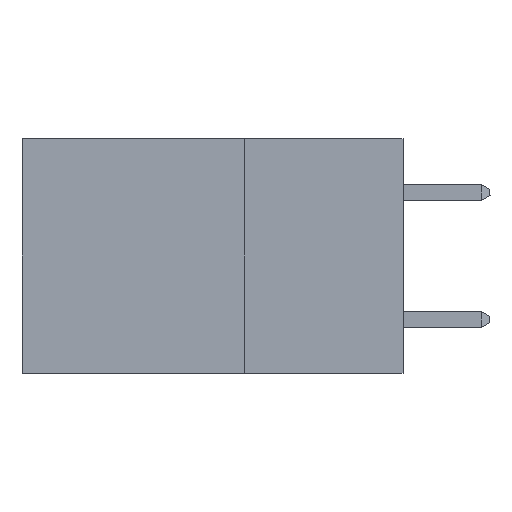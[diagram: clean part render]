
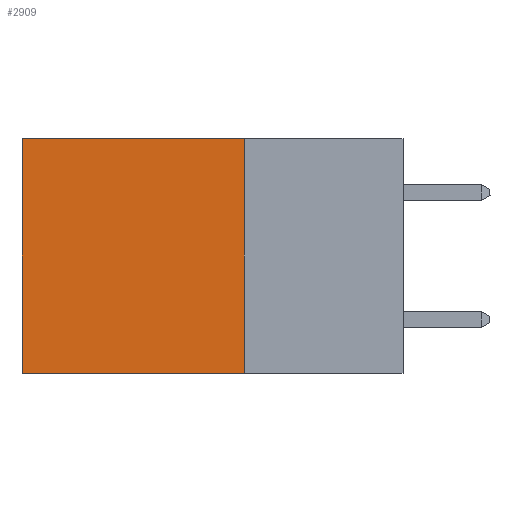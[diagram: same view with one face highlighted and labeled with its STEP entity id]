
A CAD part, left-side view. The second image highlights one B-rep face of the part: STEP entity #2909.
In plain terms, the highlighted planar face has unit normal (-1, 0, 0).
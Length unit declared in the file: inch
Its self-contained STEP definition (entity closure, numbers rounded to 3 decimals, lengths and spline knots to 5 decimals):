
#186 = DIRECTION ( 'NONE',  ( 0., 1., 0. ) ) ;
#631 = CARTESIAN_POINT ( 'NONE',  ( 0.2875, 0.25, -0.37 ) ) ;
#1118 = DIRECTION ( 'NONE',  ( 0., 0., -1. ) ) ;
#1635 = VECTOR ( 'NONE', #1118, 39.37008 ) ;
#1715 = EDGE_CURVE ( 'NONE', #31830, #31870, #19804, .T. ) ;
#2531 = VECTOR ( 'NONE', #186, 39.37008 ) ;
#2909 = ADVANCED_FACE ( 'NONE', ( #10531 ), #28943, .F. ) ;
#6049 = EDGE_LOOP ( 'NONE', ( #33644, #36590, #27035, #14759 ) ) ;
#6142 = CARTESIAN_POINT ( 'NONE',  ( 0.2875, 0.25, -0.37 ) ) ;
#6373 = CARTESIAN_POINT ( 'NONE',  ( 0.2875, 0.6, -0.37 ) ) ;
#8008 = DIRECTION ( 'NONE',  ( 0., 0., -1. ) ) ;
#8858 = VERTEX_POINT ( 'NONE', #20778 ) ;
#10531 = FACE_OUTER_BOUND ( 'NONE', #6049, .T. ) ;
#11165 = DIRECTION ( 'NONE',  ( 0., 1., 0. ) ) ;
#12763 = LINE ( 'NONE', #15657, #29853 ) ;
#14759 = ORIENTED_EDGE ( 'NONE', *, *, #36921, .T. ) ;
#15657 = CARTESIAN_POINT ( 'NONE',  ( 0.2875, 0.25, 0. ) ) ;
#17500 = LINE ( 'NONE', #31700, #34901 ) ;
#19373 = LINE ( 'NONE', #36287, #1635 ) ;
#19381 = CARTESIAN_POINT ( 'NONE',  ( 0.2875, 0.25, 0. ) ) ;
#19804 = LINE ( 'NONE', #6142, #2531 ) ;
#20778 = CARTESIAN_POINT ( 'NONE',  ( 0.2875, 0.6, 0. ) ) ;
#22239 = DIRECTION ( 'NONE',  ( 1., 0., 0. ) ) ;
#27035 = ORIENTED_EDGE ( 'NONE', *, *, #34695, .F. ) ;
#28904 = CARTESIAN_POINT ( 'NONE',  ( 0.2875, 0.25, 0. ) ) ;
#28943 = PLANE ( 'NONE',  #34511 ) ;
#29839 = DIRECTION ( 'NONE',  ( 0., 0., -1. ) ) ;
#29853 = VECTOR ( 'NONE', #29839, 39.37008 ) ;
#29951 = VERTEX_POINT ( 'NONE', #28904 ) ;
#31700 = CARTESIAN_POINT ( 'NONE',  ( 0.2875, 0.25, 0. ) ) ;
#31830 = VERTEX_POINT ( 'NONE', #631 ) ;
#31870 = VERTEX_POINT ( 'NONE', #6373 ) ;
#33644 = ORIENTED_EDGE ( 'NONE', *, *, #34384, .T. ) ;
#34384 = EDGE_CURVE ( 'NONE', #8858, #31870, #19373, .T. ) ;
#34511 = AXIS2_PLACEMENT_3D ( 'NONE', #19381, #22239, #8008 ) ;
#34695 = EDGE_CURVE ( 'NONE', #29951, #31830, #12763, .T. ) ;
#34901 = VECTOR ( 'NONE', #11165, 39.37008 ) ;
#36287 = CARTESIAN_POINT ( 'NONE',  ( 0.2875, 0.6, 0. ) ) ;
#36590 = ORIENTED_EDGE ( 'NONE', *, *, #1715, .F. ) ;
#36921 = EDGE_CURVE ( 'NONE', #29951, #8858, #17500, .T. ) ;
